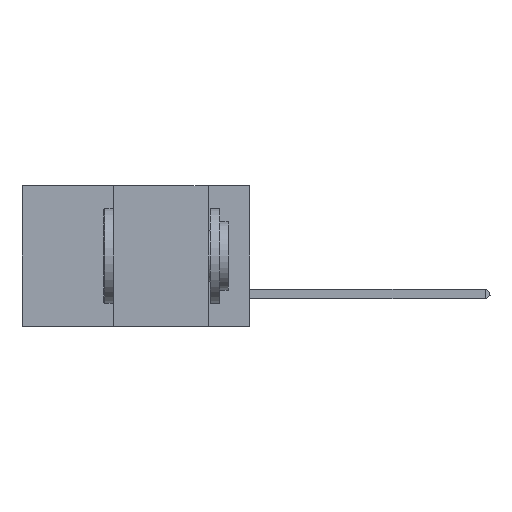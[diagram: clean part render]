
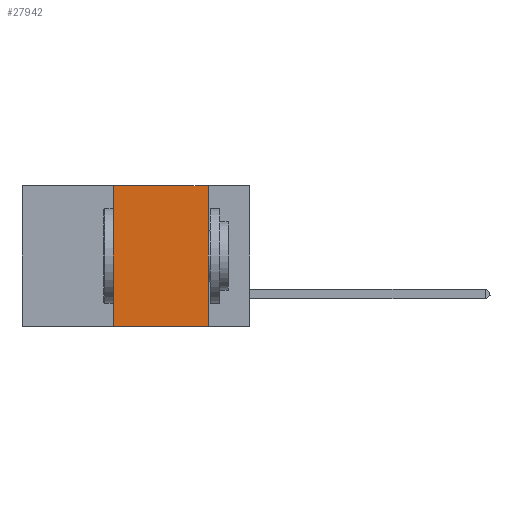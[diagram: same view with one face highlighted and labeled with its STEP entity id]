
A CAD part, left-side view. The second image highlights one B-rep face of the part: STEP entity #27942.
In plain terms, the highlighted planar face has unit normal (-1, 0, 0).
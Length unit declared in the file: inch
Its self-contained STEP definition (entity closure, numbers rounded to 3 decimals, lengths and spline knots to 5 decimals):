
#1099 = EDGE_CURVE ( 'NONE', #31616, #9346, #15302, .T. ) ;
#1476 = LINE ( 'NONE', #14564, #23840 ) ;
#1482 = PLANE ( 'NONE',  #4403 ) ;
#1947 = ORIENTED_EDGE ( 'NONE', *, *, #24733, .T. ) ;
#2596 = DIRECTION ( 'NONE',  ( 0., 0., 1. ) ) ;
#3389 = DIRECTION ( 'NONE',  ( 0., -1., 0. ) ) ;
#4403 = AXIS2_PLACEMENT_3D ( 'NONE', #26937, #29661, #29777 ) ;
#5596 = ORIENTED_EDGE ( 'NONE', *, *, #1099, .F. ) ;
#6551 = DIRECTION ( 'NONE',  ( 0., 0., -1. ) ) ;
#6787 = CARTESIAN_POINT ( 'NONE',  ( 0., 0.11, 0. ) ) ;
#8703 = EDGE_CURVE ( 'NONE', #9346, #22339, #1476, .T. ) ;
#9346 = VERTEX_POINT ( 'NONE', #17155 ) ;
#13002 = FACE_OUTER_BOUND ( 'NONE', #33411, .T. ) ;
#13166 = CARTESIAN_POINT ( 'NONE',  ( 0., 0.36, 0. ) ) ;
#14564 = CARTESIAN_POINT ( 'NONE',  ( 0., 0.6, 0. ) ) ;
#15302 = LINE ( 'NONE', #13166, #20879 ) ;
#17155 = CARTESIAN_POINT ( 'NONE',  ( 0., 0.36, 0. ) ) ;
#20485 = VECTOR ( 'NONE', #6551, 39.37008 ) ;
#20879 = VECTOR ( 'NONE', #2596, 39.37008 ) ;
#21814 = ORIENTED_EDGE ( 'NONE', *, *, #23604, .F. ) ;
#22171 = LINE ( 'NONE', #24984, #27697 ) ;
#22339 = VERTEX_POINT ( 'NONE', #6787 ) ;
#22894 = CARTESIAN_POINT ( 'NONE',  ( 0., 0.11, 0. ) ) ;
#23341 = CARTESIAN_POINT ( 'NONE',  ( 0., 0.11, -0.37 ) ) ;
#23604 = EDGE_CURVE ( 'NONE', #22339, #24906, #26908, .T. ) ;
#23840 = VECTOR ( 'NONE', #3389, 39.37008 ) ;
#24733 = EDGE_CURVE ( 'NONE', #31616, #24906, #22171, .T. ) ;
#24906 = VERTEX_POINT ( 'NONE', #23341 ) ;
#24984 = CARTESIAN_POINT ( 'NONE',  ( 0., 0.6, -0.37 ) ) ;
#26908 = LINE ( 'NONE', #22894, #20485 ) ;
#26937 = CARTESIAN_POINT ( 'NONE',  ( 0., 0.6, 0. ) ) ;
#27697 = VECTOR ( 'NONE', #33517, 39.37008 ) ;
#27862 = ORIENTED_EDGE ( 'NONE', *, *, #8703, .F. ) ;
#27942 = ADVANCED_FACE ( 'NONE', ( #13002 ), #1482, .F. ) ;
#29661 = DIRECTION ( 'NONE',  ( 1., 0., 0. ) ) ;
#29777 = DIRECTION ( 'NONE',  ( 0., 0., -1. ) ) ;
#30684 = CARTESIAN_POINT ( 'NONE',  ( 0., 0.36, -0.37 ) ) ;
#31616 = VERTEX_POINT ( 'NONE', #30684 ) ;
#33411 = EDGE_LOOP ( 'NONE', ( #21814, #27862, #5596, #1947 ) ) ;
#33517 = DIRECTION ( 'NONE',  ( 0., -1., 0. ) ) ;
